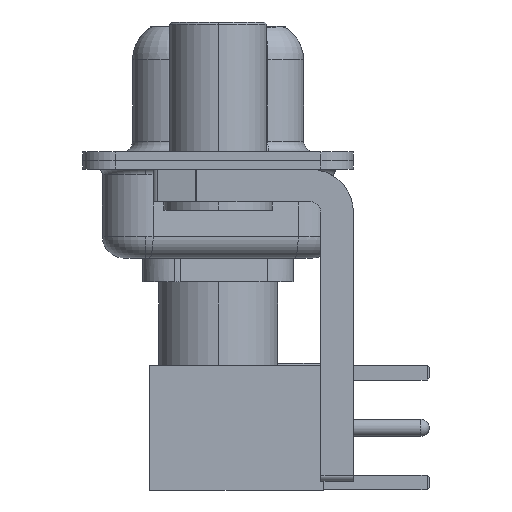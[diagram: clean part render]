
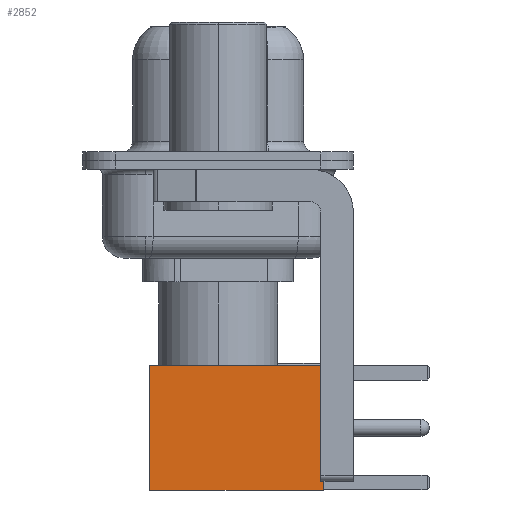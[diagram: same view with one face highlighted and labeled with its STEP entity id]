
A CAD part, left-side view. The second image highlights one B-rep face of the part: STEP entity #2852.
In plain terms, the highlighted face is planar.
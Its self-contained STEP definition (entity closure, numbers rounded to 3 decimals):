
#500 = AXIS2_PLACEMENT_3D ( 'NONE', #19232, #7543, #11752 ) ;
#818 = ORIENTED_EDGE ( 'NONE', *, *, #8643, .F. ) ;
#1061 = DIRECTION ( 'NONE',  ( 0., 0., -1. ) ) ;
#1071 = EDGE_LOOP ( 'NONE', ( #22328, #12012, #3889, #818 ) ) ;
#2103 = CARTESIAN_POINT ( 'NONE',  ( 2.875, 2.875, 0. ) ) ;
#2252 = FACE_OUTER_BOUND ( 'NONE', #1071, .T. ) ;
#2760 = LINE ( 'NONE', #28910, #2810 ) ;
#2810 = VECTOR ( 'NONE', #7586, 1000. ) ;
#2852 = ADVANCED_FACE ( 'NONE', ( #2252 ), #12074, .T. ) ;
#3889 = ORIENTED_EDGE ( 'NONE', *, *, #15123, .F. ) ;
#3966 = EDGE_CURVE ( 'NONE', #20309, #9052, #23259, .T. ) ;
#3991 = DIRECTION ( 'NONE',  ( 0., 0., -1. ) ) ;
#4862 = CARTESIAN_POINT ( 'NONE',  ( -2.875, 2.875, 8. ) ) ;
#7543 = DIRECTION ( 'NONE',  ( 0., 1., 0. ) ) ;
#7586 = DIRECTION ( 'NONE',  ( -1., 0., 0. ) ) ;
#8643 = EDGE_CURVE ( 'NONE', #20309, #15951, #2760, .T. ) ;
#9052 = VERTEX_POINT ( 'NONE', #22177 ) ;
#9159 = CARTESIAN_POINT ( 'NONE',  ( 2.875, 2.875, 8. ) ) ;
#9649 = VERTEX_POINT ( 'NONE', #21722 ) ;
#10571 = LINE ( 'NONE', #13063, #27478 ) ;
#11752 = DIRECTION ( 'NONE',  ( 0., 0., 1. ) ) ;
#12012 = ORIENTED_EDGE ( 'NONE', *, *, #18814, .T. ) ;
#12074 = PLANE ( 'NONE',  #500 ) ;
#13063 = CARTESIAN_POINT ( 'NONE',  ( -2.875, 2.875, 0. ) ) ;
#15123 = EDGE_CURVE ( 'NONE', #15951, #9649, #10571, .T. ) ;
#15746 = LINE ( 'NONE', #18079, #24093 ) ;
#15951 = VERTEX_POINT ( 'NONE', #4862 ) ;
#18079 = CARTESIAN_POINT ( 'NONE',  ( 0., 2.875, 0. ) ) ;
#18814 = EDGE_CURVE ( 'NONE', #9052, #9649, #15746, .T. ) ;
#19232 = CARTESIAN_POINT ( 'NONE',  ( 2.875, 2.875, 0. ) ) ;
#20309 = VERTEX_POINT ( 'NONE', #9159 ) ;
#21722 = CARTESIAN_POINT ( 'NONE',  ( -2.875, 2.875, 0. ) ) ;
#22177 = CARTESIAN_POINT ( 'NONE',  ( 2.875, 2.875, 0. ) ) ;
#22328 = ORIENTED_EDGE ( 'NONE', *, *, #3966, .T. ) ;
#22712 = VECTOR ( 'NONE', #3991, 1000. ) ;
#23020 = DIRECTION ( 'NONE',  ( -1., 0., 0. ) ) ;
#23259 = LINE ( 'NONE', #2103, #22712 ) ;
#24093 = VECTOR ( 'NONE', #23020, 1000. ) ;
#27478 = VECTOR ( 'NONE', #1061, 1000. ) ;
#28910 = CARTESIAN_POINT ( 'NONE',  ( 0., 2.875, 8. ) ) ;
